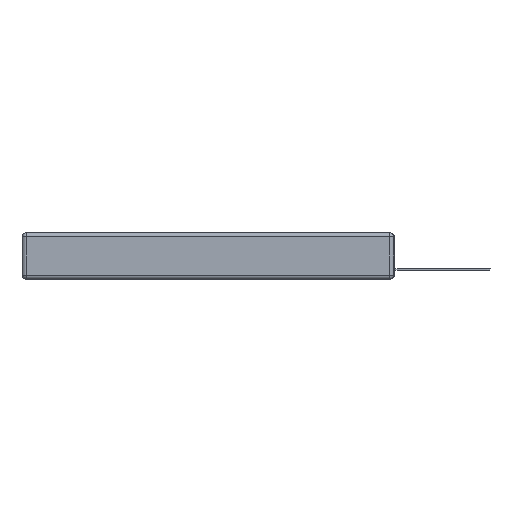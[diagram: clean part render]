
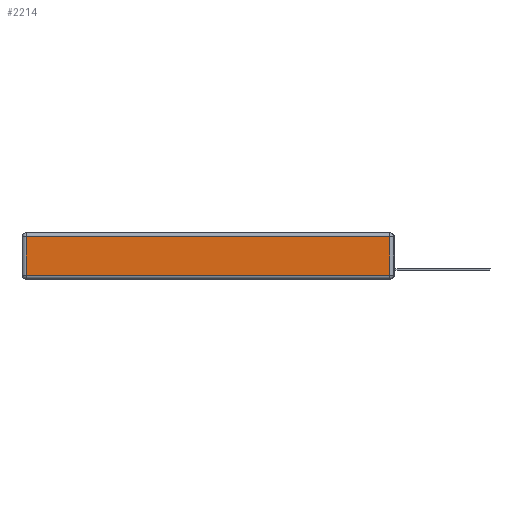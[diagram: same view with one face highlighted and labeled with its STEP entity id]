
A CAD part, left-side view. The second image highlights one B-rep face of the part: STEP entity #2214.
In plain terms, the highlighted planar face has unit normal (-1, 0, 0).
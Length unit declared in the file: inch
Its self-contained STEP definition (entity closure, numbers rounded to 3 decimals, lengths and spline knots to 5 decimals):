
#665 = EDGE_CURVE ( 'NONE', #5980, #4214, #2658, .T. ) ;
#741 = VECTOR ( 'NONE', #8393, 39.37008 ) ;
#2162 = VECTOR ( 'NONE', #15701, 39.37008 ) ;
#2214 = ADVANCED_FACE ( 'NONE', ( #6521 ), #12141, .T. ) ;
#2286 = DIRECTION ( 'NONE',  ( -1., 0., 0. ) ) ;
#2480 = CARTESIAN_POINT ( 'NONE',  ( 0., 0., -0.313 ) ) ;
#2658 = LINE ( 'NONE', #2480, #15374 ) ;
#3568 = CARTESIAN_POINT ( 'NONE',  ( 0., 0., -0.343 ) ) ;
#3690 = EDGE_LOOP ( 'NONE', ( #6109, #6738, #9945, #5122 ) ) ;
#4214 = VERTEX_POINT ( 'NONE', #12982 ) ;
#4273 = CARTESIAN_POINT ( 'NONE',  ( 0., 0.03, -0.343 ) ) ;
#5122 = ORIENTED_EDGE ( 'NONE', *, *, #15296, .T. ) ;
#5542 = CARTESIAN_POINT ( 'NONE',  ( 0., 0.03, -0.03 ) ) ;
#5980 = VERTEX_POINT ( 'NONE', #14971 ) ;
#6109 = ORIENTED_EDGE ( 'NONE', *, *, #665, .T. ) ;
#6521 = FACE_OUTER_BOUND ( 'NONE', #3690, .T. ) ;
#6738 = ORIENTED_EDGE ( 'NONE', *, *, #11248, .T. ) ;
#6896 = DIRECTION ( 'NONE',  ( 0., -1., 0. ) ) ;
#6907 = EDGE_CURVE ( 'NONE', #7985, #11047, #13634, .T. ) ;
#6921 = LINE ( 'NONE', #16773, #741 ) ;
#7985 = VERTEX_POINT ( 'NONE', #5542 ) ;
#8393 = DIRECTION ( 'NONE',  ( 0., 0., -1. ) ) ;
#9945 = ORIENTED_EDGE ( 'NONE', *, *, #6907, .T. ) ;
#10054 = AXIS2_PLACEMENT_3D ( 'NONE', #3568, #2286, #11955 ) ;
#10067 = LINE ( 'NONE', #4273, #2162 ) ;
#11047 = VERTEX_POINT ( 'NONE', #12112 ) ;
#11248 = EDGE_CURVE ( 'NONE', #4214, #7985, #10067, .T. ) ;
#11955 = DIRECTION ( 'NONE',  ( 0., 0., 1. ) ) ;
#12112 = CARTESIAN_POINT ( 'NONE',  ( 0., 2.72, -0.03 ) ) ;
#12141 = PLANE ( 'NONE',  #10054 ) ;
#12982 = CARTESIAN_POINT ( 'NONE',  ( 0., 0.03, -0.313 ) ) ;
#13634 = LINE ( 'NONE', #16587, #17913 ) ;
#14971 = CARTESIAN_POINT ( 'NONE',  ( 0., 2.72, -0.313 ) ) ;
#15296 = EDGE_CURVE ( 'NONE', #11047, #5980, #6921, .T. ) ;
#15374 = VECTOR ( 'NONE', #6896, 39.37008 ) ;
#15701 = DIRECTION ( 'NONE',  ( 0., 0., 1. ) ) ;
#16587 = CARTESIAN_POINT ( 'NONE',  ( 0., 2.75, -0.03 ) ) ;
#16773 = CARTESIAN_POINT ( 'NONE',  ( 0., 2.72, -0.343 ) ) ;
#17913 = VECTOR ( 'NONE', #18030, 39.37008 ) ;
#18030 = DIRECTION ( 'NONE',  ( 0., 1., 0. ) ) ;
